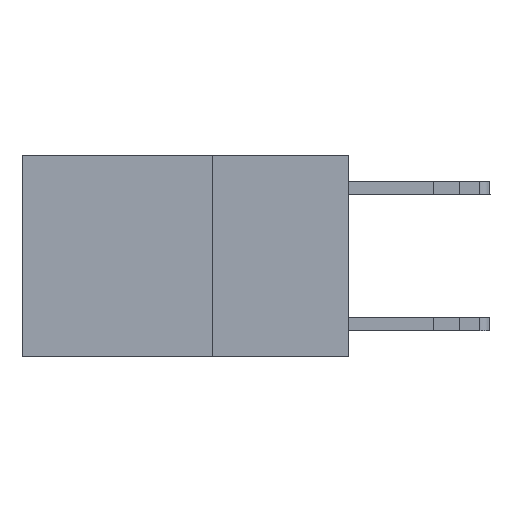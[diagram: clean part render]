
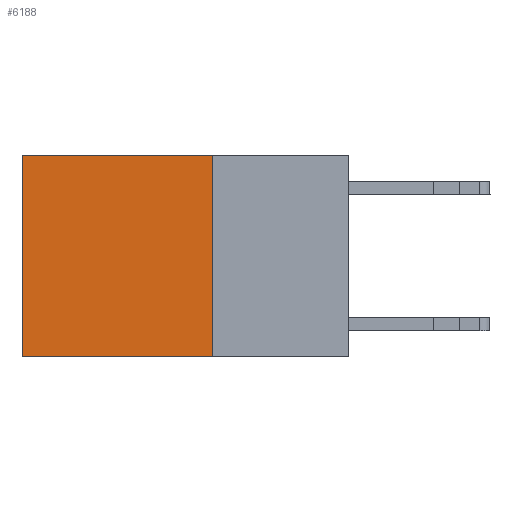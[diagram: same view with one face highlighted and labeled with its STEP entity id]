
A CAD part, left-side view. The second image highlights one B-rep face of the part: STEP entity #6188.
In plain terms, the highlighted planar face has unit normal (-1, 0, 0).
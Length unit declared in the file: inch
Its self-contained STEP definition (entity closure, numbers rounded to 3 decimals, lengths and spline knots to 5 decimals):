
#53 = LINE ( 'NONE', #2537, #12061 ) ;
#156 = DIRECTION ( 'NONE',  ( 0., 1., 0. ) ) ;
#761 = EDGE_LOOP ( 'NONE', ( #7560, #16046, #10633, #16338 ) ) ;
#1886 = LINE ( 'NONE', #14722, #12308 ) ;
#2422 = EDGE_CURVE ( 'NONE', #4334, #9655, #11866, .T. ) ;
#2537 = CARTESIAN_POINT ( 'NONE',  ( 0.2625, 0.6, 0. ) ) ;
#4334 = VERTEX_POINT ( 'NONE', #10750 ) ;
#6188 = ADVANCED_FACE ( 'NONE', ( #15138 ), #12205, .F. ) ;
#6542 = CARTESIAN_POINT ( 'NONE',  ( 0.2625, 0.6, -0.37 ) ) ;
#6979 = CARTESIAN_POINT ( 'NONE',  ( 0.2625, 0.25, 0. ) ) ;
#7482 = VERTEX_POINT ( 'NONE', #9199 ) ;
#7516 = DIRECTION ( 'NONE',  ( 0., 1., 0. ) ) ;
#7560 = ORIENTED_EDGE ( 'NONE', *, *, #13153, .T. ) ;
#8190 = CARTESIAN_POINT ( 'NONE',  ( 0.2625, 0.25, -0.37 ) ) ;
#8376 = VERTEX_POINT ( 'NONE', #15875 ) ;
#8467 = AXIS2_PLACEMENT_3D ( 'NONE', #6979, #12128, #13592 ) ;
#8736 = CARTESIAN_POINT ( 'NONE',  ( 0.2625, 0.25, 0. ) ) ;
#9199 = CARTESIAN_POINT ( 'NONE',  ( 0.2625, 0.6, 0. ) ) ;
#9481 = VECTOR ( 'NONE', #7516, 39.37008 ) ;
#9655 = VERTEX_POINT ( 'NONE', #6542 ) ;
#9830 = LINE ( 'NONE', #8736, #9481 ) ;
#10571 = EDGE_CURVE ( 'NONE', #8376, #4334, #1886, .T. ) ;
#10633 = ORIENTED_EDGE ( 'NONE', *, *, #10571, .F. ) ;
#10750 = CARTESIAN_POINT ( 'NONE',  ( 0.2625, 0.25, -0.37 ) ) ;
#10828 = DIRECTION ( 'NONE',  ( 0., 0., -1. ) ) ;
#11842 = DIRECTION ( 'NONE',  ( 0., 0., -1. ) ) ;
#11866 = LINE ( 'NONE', #8190, #16092 ) ;
#12061 = VECTOR ( 'NONE', #11842, 39.37008 ) ;
#12128 = DIRECTION ( 'NONE',  ( 1., 0., 0. ) ) ;
#12205 = PLANE ( 'NONE',  #8467 ) ;
#12308 = VECTOR ( 'NONE', #10828, 39.37008 ) ;
#13153 = EDGE_CURVE ( 'NONE', #7482, #9655, #53, .T. ) ;
#13592 = DIRECTION ( 'NONE',  ( 0., 0., -1. ) ) ;
#13963 = EDGE_CURVE ( 'NONE', #8376, #7482, #9830, .T. ) ;
#14722 = CARTESIAN_POINT ( 'NONE',  ( 0.2625, 0.25, 0. ) ) ;
#15138 = FACE_OUTER_BOUND ( 'NONE', #761, .T. ) ;
#15875 = CARTESIAN_POINT ( 'NONE',  ( 0.2625, 0.25, 0. ) ) ;
#16046 = ORIENTED_EDGE ( 'NONE', *, *, #2422, .F. ) ;
#16092 = VECTOR ( 'NONE', #156, 39.37008 ) ;
#16338 = ORIENTED_EDGE ( 'NONE', *, *, #13963, .T. ) ;
